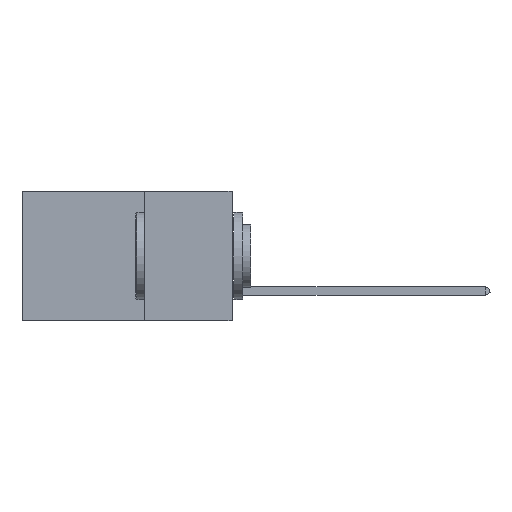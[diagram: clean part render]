
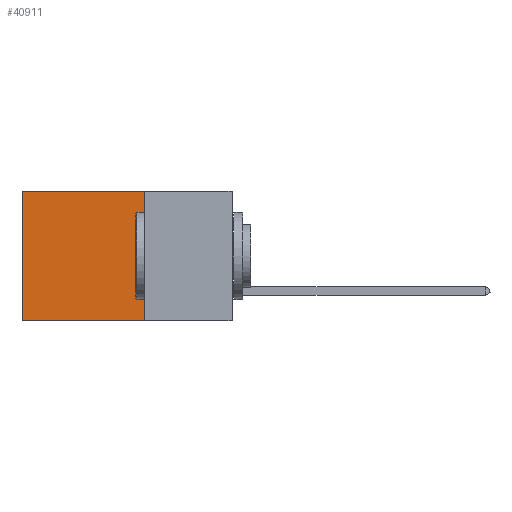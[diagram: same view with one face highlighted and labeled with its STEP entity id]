
A CAD part, left-side view. The second image highlights one B-rep face of the part: STEP entity #40911.
In plain terms, the highlighted planar face has unit normal (-1, 0, 0).
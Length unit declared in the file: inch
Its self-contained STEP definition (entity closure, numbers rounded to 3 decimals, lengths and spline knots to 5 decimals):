
#2971 = LINE ( 'NONE', #40567, #14272 ) ;
#3947 = LINE ( 'NONE', #24174, #32970 ) ;
#4404 = ORIENTED_EDGE ( 'NONE', *, *, #16501, .F. ) ;
#4676 = CARTESIAN_POINT ( 'NONE',  ( 0.2875, 0.25, 0. ) ) ;
#5137 = LINE ( 'NONE', #22003, #7296 ) ;
#5290 = DIRECTION ( 'NONE',  ( 0., 1., 0. ) ) ;
#5320 = EDGE_CURVE ( 'NONE', #10436, #33854, #3947, .T. ) ;
#5382 = CARTESIAN_POINT ( 'NONE',  ( 0.2875, 0.6, -0.37 ) ) ;
#7296 = VECTOR ( 'NONE', #5290, 39.37008 ) ;
#8011 = DIRECTION ( 'NONE',  ( 1., 0., 0. ) ) ;
#8195 = AXIS2_PLACEMENT_3D ( 'NONE', #4676, #8011, #13843 ) ;
#9968 = CARTESIAN_POINT ( 'NONE',  ( 0.2875, 0.25, 0. ) ) ;
#10436 = VERTEX_POINT ( 'NONE', #32346 ) ;
#11747 = PLANE ( 'NONE',  #8195 ) ;
#12122 = DIRECTION ( 'NONE',  ( 0., 0., -1. ) ) ;
#13709 = FACE_OUTER_BOUND ( 'NONE', #25429, .T. ) ;
#13843 = DIRECTION ( 'NONE',  ( 0., 0., -1. ) ) ;
#14272 = VECTOR ( 'NONE', #26806, 39.37008 ) ;
#16501 = EDGE_CURVE ( 'NONE', #27247, #31351, #40061, .T. ) ;
#19009 = ORIENTED_EDGE ( 'NONE', *, *, #5320, .T. ) ;
#22003 = CARTESIAN_POINT ( 'NONE',  ( 0.2875, 0.25, -0.37 ) ) ;
#22968 = EDGE_CURVE ( 'NONE', #27247, #10436, #2971, .T. ) ;
#24174 = CARTESIAN_POINT ( 'NONE',  ( 0.2875, 0.6, 0. ) ) ;
#24406 = VECTOR ( 'NONE', #44501, 39.37008 ) ;
#25242 = ORIENTED_EDGE ( 'NONE', *, *, #40594, .F. ) ;
#25429 = EDGE_LOOP ( 'NONE', ( #19009, #25242, #4404, #36031 ) ) ;
#26806 = DIRECTION ( 'NONE',  ( 0., 1., 0. ) ) ;
#27247 = VERTEX_POINT ( 'NONE', #39266 ) ;
#31351 = VERTEX_POINT ( 'NONE', #33556 ) ;
#32346 = CARTESIAN_POINT ( 'NONE',  ( 0.2875, 0.6, 0. ) ) ;
#32970 = VECTOR ( 'NONE', #12122, 39.37008 ) ;
#33556 = CARTESIAN_POINT ( 'NONE',  ( 0.2875, 0.25, -0.37 ) ) ;
#33854 = VERTEX_POINT ( 'NONE', #5382 ) ;
#36031 = ORIENTED_EDGE ( 'NONE', *, *, #22968, .T. ) ;
#39266 = CARTESIAN_POINT ( 'NONE',  ( 0.2875, 0.25, 0. ) ) ;
#40061 = LINE ( 'NONE', #9968, #24406 ) ;
#40567 = CARTESIAN_POINT ( 'NONE',  ( 0.2875, 0.25, 0. ) ) ;
#40594 = EDGE_CURVE ( 'NONE', #31351, #33854, #5137, .T. ) ;
#40911 = ADVANCED_FACE ( 'NONE', ( #13709 ), #11747, .F. ) ;
#44501 = DIRECTION ( 'NONE',  ( 0., 0., -1. ) ) ;
